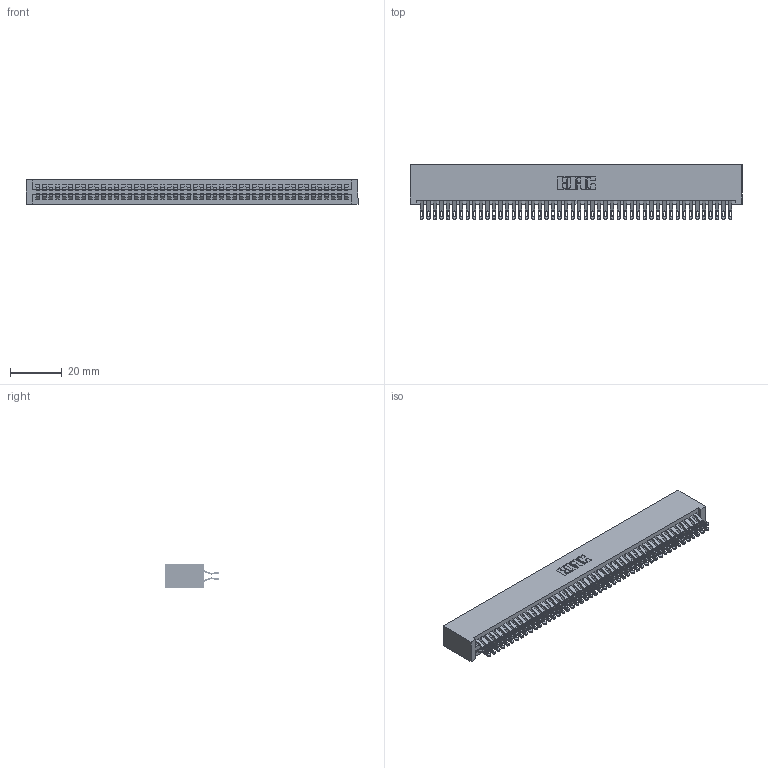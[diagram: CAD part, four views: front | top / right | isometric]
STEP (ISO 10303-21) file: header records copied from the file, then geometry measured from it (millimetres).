
FILE_DESCRIPTION (( 'STEP AP203' ), '1' );
FILE_NAME ('345-096-555-201.STEP', '2019-11-02T08:36:27', ( '' ), ( '' ), 'SwSTEP 2.0', 'SolidWorks 2016', '' );
FILE_SCHEMA (( 'CONFIG_CONTROL_DESIGN' ));
Length unit declared in the file: inch
Products named in the file (3): 345-292-001_555 Tail; 345-096-555-201; 345 Part_No Mounting Lugs
Assembly tree (97 placements, depth 2):
  345-096-555-201
    345 Part_No Mounting Lugs
    345-292-001_555 Tail  x96
Bounding box: 128.52 x 21.13 x 9.4 mm (x, y, z)
Volume: 13435 mm3; surface area: 21247.2 mm2
Topology: 97 solids, 97 shells, 5494 faces, 17309 edges, 11538 vertices
Faces by surface type: plane 3052, cylinder 2442
Entity records: 36903 total; most frequent: CARTESIAN_POINT 6214, ORIENTED_EDGE 6118, DIRECTION 5435, EDGE_CURVE 3059, VECTOR 2723, LINE 2723, VERTEX_POINT 2038, AXIS2_PLACEMENT_3D 1356
